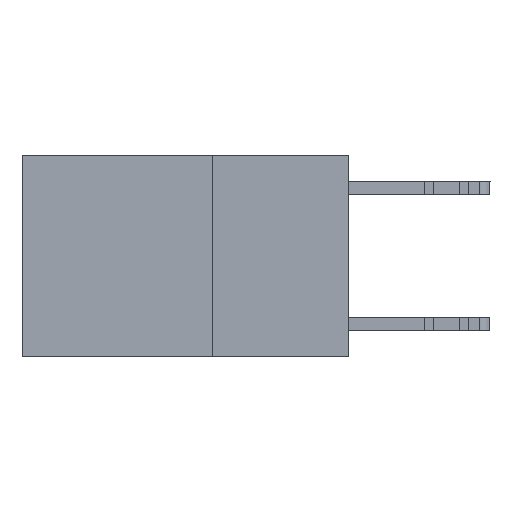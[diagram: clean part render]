
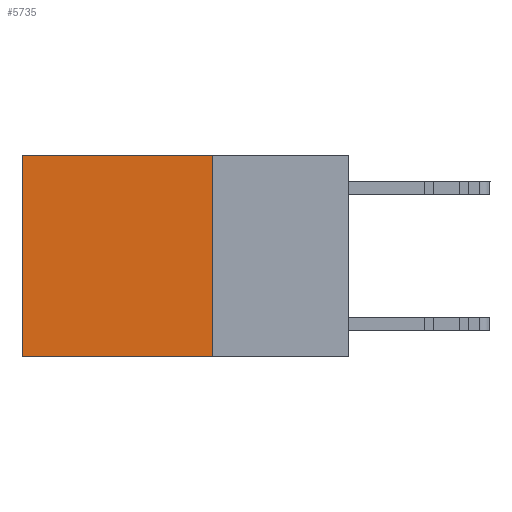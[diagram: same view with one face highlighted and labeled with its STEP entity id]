
A CAD part, left-side view. The second image highlights one B-rep face of the part: STEP entity #5735.
In plain terms, the highlighted planar face has unit normal (-1, 0, 0).
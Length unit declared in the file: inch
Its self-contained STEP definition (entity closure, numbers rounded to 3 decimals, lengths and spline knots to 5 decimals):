
#459 = CARTESIAN_POINT ( 'NONE',  ( 0.2625, 0.25, 0. ) ) ;
#1066 = VECTOR ( 'NONE', #4412, 39.37008 ) ;
#4412 = DIRECTION ( 'NONE',  ( 0., 0., -1. ) ) ;
#4988 = DIRECTION ( 'NONE',  ( 0., 0., -1. ) ) ;
#5735 = ADVANCED_FACE ( 'NONE', ( #23916 ), #12052, .F. ) ;
#6865 = CARTESIAN_POINT ( 'NONE',  ( 0.2625, 0.25, 0. ) ) ;
#7812 = VECTOR ( 'NONE', #12391, 39.37008 ) ;
#8667 = ORIENTED_EDGE ( 'NONE', *, *, #12656, .F. ) ;
#9390 = ORIENTED_EDGE ( 'NONE', *, *, #20898, .F. ) ;
#9695 = DIRECTION ( 'NONE',  ( 1., 0., 0. ) ) ;
#9931 = LINE ( 'NONE', #14642, #26042 ) ;
#11185 = CARTESIAN_POINT ( 'NONE',  ( 0.2625, 0.25, -0.37 ) ) ;
#11217 = EDGE_CURVE ( 'NONE', #14493, #21031, #21165, .T. ) ;
#12052 = PLANE ( 'NONE',  #26358 ) ;
#12391 = DIRECTION ( 'NONE',  ( 0., 0., -1. ) ) ;
#12471 = CARTESIAN_POINT ( 'NONE',  ( 0.2625, 0.25, 0. ) ) ;
#12656 = EDGE_CURVE ( 'NONE', #24467, #21031, #9931, .T. ) ;
#13565 = EDGE_LOOP ( 'NONE', ( #30488, #8667, #9390, #24269 ) ) ;
#14493 = VERTEX_POINT ( 'NONE', #23760 ) ;
#14642 = CARTESIAN_POINT ( 'NONE',  ( 0.2625, 0.25, -0.37 ) ) ;
#15961 = DIRECTION ( 'NONE',  ( 0., 1., 0. ) ) ;
#16497 = VECTOR ( 'NONE', #15961, 39.37008 ) ;
#16830 = DIRECTION ( 'NONE',  ( 0., 1., 0. ) ) ;
#19891 = LINE ( 'NONE', #459, #7812 ) ;
#20898 = EDGE_CURVE ( 'NONE', #27812, #24467, #19891, .T. ) ;
#21031 = VERTEX_POINT ( 'NONE', #29560 ) ;
#21165 = LINE ( 'NONE', #30685, #1066 ) ;
#21594 = CARTESIAN_POINT ( 'NONE',  ( 0.2625, 0.25, 0. ) ) ;
#23760 = CARTESIAN_POINT ( 'NONE',  ( 0.2625, 0.6, 0. ) ) ;
#23916 = FACE_OUTER_BOUND ( 'NONE', #13565, .T. ) ;
#24269 = ORIENTED_EDGE ( 'NONE', *, *, #25574, .T. ) ;
#24467 = VERTEX_POINT ( 'NONE', #11185 ) ;
#25574 = EDGE_CURVE ( 'NONE', #27812, #14493, #28302, .T. ) ;
#26042 = VECTOR ( 'NONE', #16830, 39.37008 ) ;
#26358 = AXIS2_PLACEMENT_3D ( 'NONE', #21594, #9695, #4988 ) ;
#27812 = VERTEX_POINT ( 'NONE', #12471 ) ;
#28302 = LINE ( 'NONE', #6865, #16497 ) ;
#29560 = CARTESIAN_POINT ( 'NONE',  ( 0.2625, 0.6, -0.37 ) ) ;
#30488 = ORIENTED_EDGE ( 'NONE', *, *, #11217, .T. ) ;
#30685 = CARTESIAN_POINT ( 'NONE',  ( 0.2625, 0.6, 0. ) ) ;
